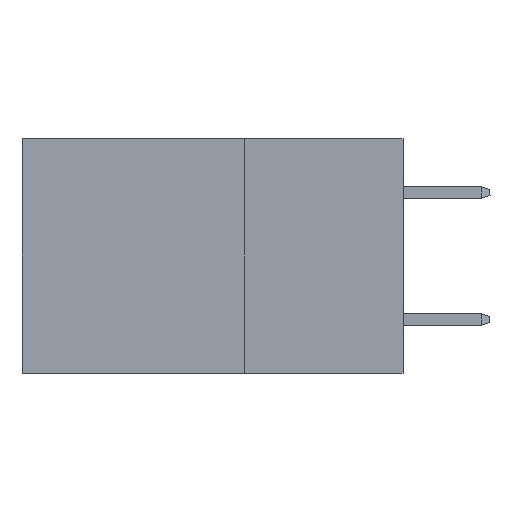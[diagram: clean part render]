
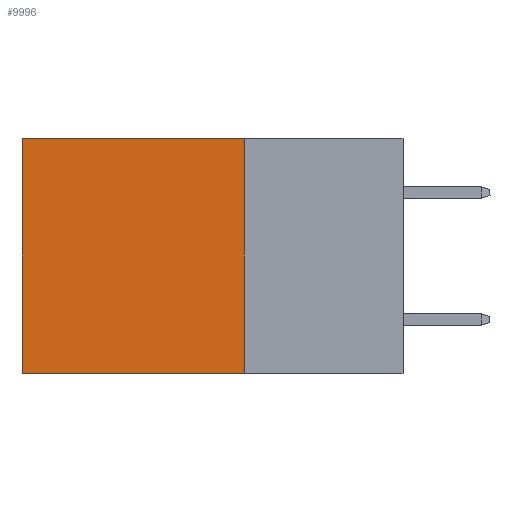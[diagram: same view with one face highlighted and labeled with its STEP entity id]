
A CAD part, left-side view. The second image highlights one B-rep face of the part: STEP entity #9996.
In plain terms, the highlighted planar face has unit normal (-1, 0, 0).
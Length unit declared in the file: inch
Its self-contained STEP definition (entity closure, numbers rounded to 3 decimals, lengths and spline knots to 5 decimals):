
#6 = CARTESIAN_POINT ( 'NONE',  ( 0.2875, 0.6, 0. ) ) ;
#1015 = CARTESIAN_POINT ( 'NONE',  ( 0.2875, 0.6, -0.37 ) ) ;
#1149 = LINE ( 'NONE', #11189, #1382 ) ;
#1382 = VECTOR ( 'NONE', #13873, 39.37008 ) ;
#1636 = DIRECTION ( 'NONE',  ( 0., 1., 0. ) ) ;
#2256 = LINE ( 'NONE', #6995, #12230 ) ;
#2575 = EDGE_LOOP ( 'NONE', ( #14522, #11389, #9680, #13048 ) ) ;
#2619 = LINE ( 'NONE', #15191, #3976 ) ;
#2732 = VECTOR ( 'NONE', #1636, 39.37008 ) ;
#2970 = CARTESIAN_POINT ( 'NONE',  ( 0.2875, 0.25, 0. ) ) ;
#3009 = EDGE_CURVE ( 'NONE', #4642, #3581, #2256, .T. ) ;
#3581 = VERTEX_POINT ( 'NONE', #1015 ) ;
#3976 = VECTOR ( 'NONE', #7615, 39.37008 ) ;
#4161 = CARTESIAN_POINT ( 'NONE',  ( 0.2875, 0.25, 0. ) ) ;
#4241 = LINE ( 'NONE', #4161, #2732 ) ;
#4642 = VERTEX_POINT ( 'NONE', #9669 ) ;
#6643 = EDGE_CURVE ( 'NONE', #14658, #13209, #4241, .T. ) ;
#6995 = CARTESIAN_POINT ( 'NONE',  ( 0.2875, 0.25, -0.37 ) ) ;
#7615 = DIRECTION ( 'NONE',  ( 0., 0., -1. ) ) ;
#7961 = DIRECTION ( 'NONE',  ( 1., 0., 0. ) ) ;
#9669 = CARTESIAN_POINT ( 'NONE',  ( 0.2875, 0.25, -0.37 ) ) ;
#9680 = ORIENTED_EDGE ( 'NONE', *, *, #13197, .F. ) ;
#9996 = ADVANCED_FACE ( 'NONE', ( #15395 ), #14151, .F. ) ;
#10590 = CARTESIAN_POINT ( 'NONE',  ( 0.2875, 0.25, 0. ) ) ;
#11189 = CARTESIAN_POINT ( 'NONE',  ( 0.2875, 0.25, 0. ) ) ;
#11389 = ORIENTED_EDGE ( 'NONE', *, *, #3009, .F. ) ;
#11956 = DIRECTION ( 'NONE',  ( 0., 1., 0. ) ) ;
#12230 = VECTOR ( 'NONE', #11956, 39.37008 ) ;
#12526 = AXIS2_PLACEMENT_3D ( 'NONE', #2970, #7961, #12921 ) ;
#12921 = DIRECTION ( 'NONE',  ( 0., 0., -1. ) ) ;
#13048 = ORIENTED_EDGE ( 'NONE', *, *, #6643, .T. ) ;
#13197 = EDGE_CURVE ( 'NONE', #14658, #4642, #1149, .T. ) ;
#13209 = VERTEX_POINT ( 'NONE', #6 ) ;
#13873 = DIRECTION ( 'NONE',  ( 0., 0., -1. ) ) ;
#14151 = PLANE ( 'NONE',  #12526 ) ;
#14522 = ORIENTED_EDGE ( 'NONE', *, *, #14577, .T. ) ;
#14577 = EDGE_CURVE ( 'NONE', #13209, #3581, #2619, .T. ) ;
#14658 = VERTEX_POINT ( 'NONE', #10590 ) ;
#15191 = CARTESIAN_POINT ( 'NONE',  ( 0.2875, 0.6, 0. ) ) ;
#15395 = FACE_OUTER_BOUND ( 'NONE', #2575, .T. ) ;
